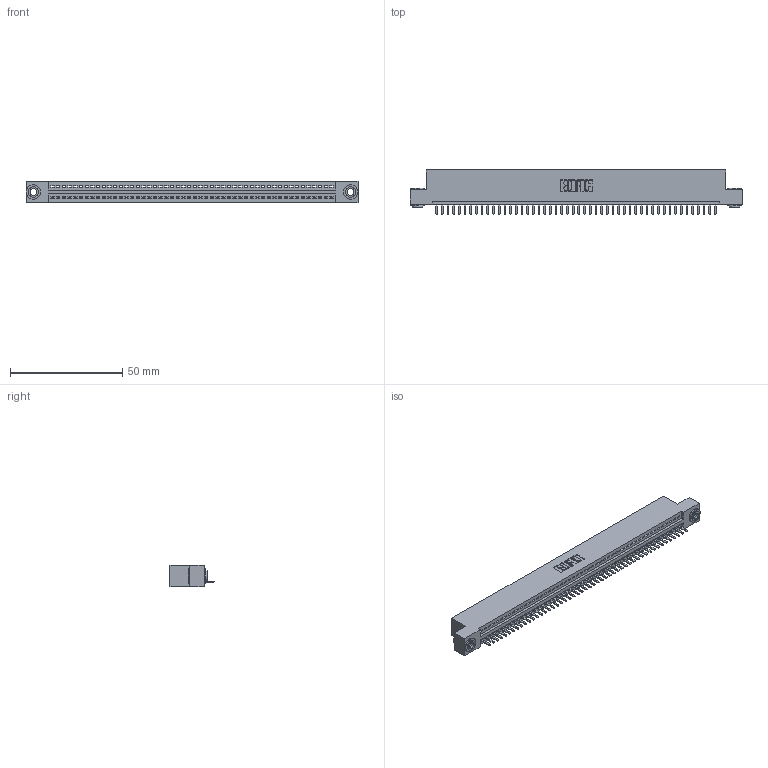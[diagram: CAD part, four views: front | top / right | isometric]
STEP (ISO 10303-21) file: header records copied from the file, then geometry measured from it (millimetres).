
FILE_DESCRIPTION (( 'STEP AP203' ), '1' );
FILE_NAME ('345-050-520-103.STEP', '2018-09-14T02:40:22', ( '' ), ( '' ), 'SwSTEP 2.0', 'SolidWorks 2016', '' );
FILE_SCHEMA (( 'CONFIG_CONTROL_DESIGN' ));
Length unit declared in the file: inch
Products named in the file (4): 345 Part_Flush Mounting Lugs - 0.156 Dia-TH; 345-292-001_345-293-120; 345-250-002_345-250-002-102; 345-050-520-103
Assembly tree (53 placements, depth 2):
  345-050-520-103
    345 Part_Flush Mounting Lugs - 0.156 Dia-TH
    345-292-001_345-293-120  x50
    345-250-002_345-250-002-102  x2
Bounding box: 148.21 x 19.68 x 9.4 mm (x, y, z)
Volume: 14018.1 mm3; surface area: 18481.5 mm2
Topology: 53 solids, 53 shells, 3264 faces, 9617 edges, 6274 vertices
Faces by surface type: plane 2190, cylinder 1066, cone 8
Entity records: 37318 total; most frequent: CARTESIAN_POINT 6453, ORIENTED_EDGE 6418, DIRECTION 5643, EDGE_CURVE 3209, VECTOR 2849, LINE 2849, VERTEX_POINT 2134, AXIS2_PLACEMENT_3D 1397
